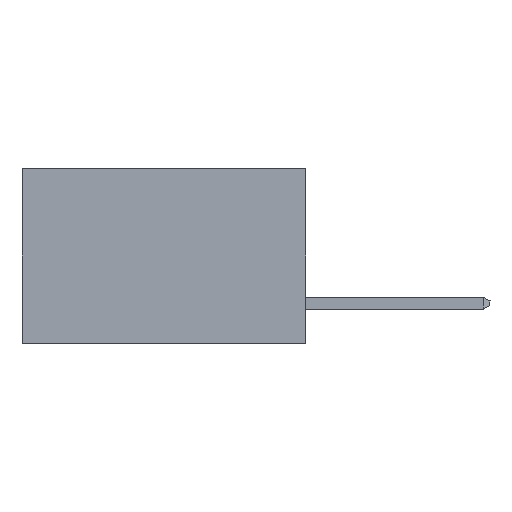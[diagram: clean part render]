
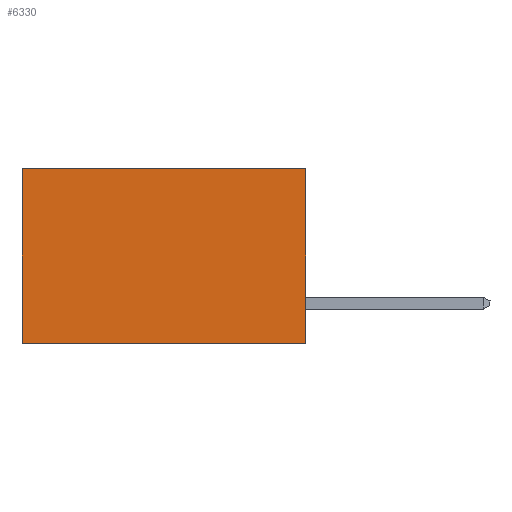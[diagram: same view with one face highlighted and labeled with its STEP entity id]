
A CAD part, left-side view. The second image highlights one B-rep face of the part: STEP entity #6330.
In plain terms, the highlighted planar face has unit normal (-1, 0, 0).
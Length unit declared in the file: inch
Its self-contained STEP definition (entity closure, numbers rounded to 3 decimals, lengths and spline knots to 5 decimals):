
#149 = DIRECTION ( 'NONE',  ( 0., 0., -1. ) ) ;
#611 = CARTESIAN_POINT ( 'NONE',  ( 0.298, 0., 0. ) ) ;
#1782 = LINE ( 'NONE', #18143, #16651 ) ;
#2880 = DIRECTION ( 'NONE',  ( 0., 0., -1. ) ) ;
#3373 = CARTESIAN_POINT ( 'NONE',  ( 0.298, 0.6, -0.37 ) ) ;
#4091 = CARTESIAN_POINT ( 'NONE',  ( 0.298, 0., 0. ) ) ;
#4401 = VERTEX_POINT ( 'NONE', #611 ) ;
#4864 = LINE ( 'NONE', #10929, #11615 ) ;
#5112 = DIRECTION ( 'NONE',  ( 0., 1., 0. ) ) ;
#5606 = CARTESIAN_POINT ( 'NONE',  ( 0.298, 0.6, 0. ) ) ;
#6330 = ADVANCED_FACE ( 'NONE', ( #14099 ), #11244, .F. ) ;
#6711 = DIRECTION ( 'NONE',  ( 0., 0., -1. ) ) ;
#6795 = CARTESIAN_POINT ( 'NONE',  ( 0.298, 0.6, 0. ) ) ;
#7055 = AXIS2_PLACEMENT_3D ( 'NONE', #4091, #17512, #149 ) ;
#7122 = EDGE_CURVE ( 'NONE', #4401, #9740, #12042, .T. ) ;
#7131 = LINE ( 'NONE', #5606, #9578 ) ;
#7983 = VECTOR ( 'NONE', #9682, 39.37008 ) ;
#8058 = VERTEX_POINT ( 'NONE', #3373 ) ;
#9578 = VECTOR ( 'NONE', #2880, 39.37008 ) ;
#9581 = ORIENTED_EDGE ( 'NONE', *, *, #7122, .T. ) ;
#9682 = DIRECTION ( 'NONE',  ( 0., 1., 0. ) ) ;
#9740 = VERTEX_POINT ( 'NONE', #6795 ) ;
#10001 = ORIENTED_EDGE ( 'NONE', *, *, #16575, .T. ) ;
#10256 = EDGE_CURVE ( 'NONE', #4401, #18579, #1782, .T. ) ;
#10929 = CARTESIAN_POINT ( 'NONE',  ( 0.298, 0., -0.37 ) ) ;
#11112 = EDGE_LOOP ( 'NONE', ( #10001, #12701, #12853, #9581 ) ) ;
#11244 = PLANE ( 'NONE',  #7055 ) ;
#11568 = EDGE_CURVE ( 'NONE', #18579, #8058, #4864, .T. ) ;
#11615 = VECTOR ( 'NONE', #5112, 39.37008 ) ;
#12042 = LINE ( 'NONE', #13852, #7983 ) ;
#12701 = ORIENTED_EDGE ( 'NONE', *, *, #11568, .F. ) ;
#12853 = ORIENTED_EDGE ( 'NONE', *, *, #10256, .F. ) ;
#13852 = CARTESIAN_POINT ( 'NONE',  ( 0.298, 0., 0. ) ) ;
#14099 = FACE_OUTER_BOUND ( 'NONE', #11112, .T. ) ;
#16575 = EDGE_CURVE ( 'NONE', #9740, #8058, #7131, .T. ) ;
#16651 = VECTOR ( 'NONE', #6711, 39.37008 ) ;
#17512 = DIRECTION ( 'NONE',  ( 1., 0., 0. ) ) ;
#18143 = CARTESIAN_POINT ( 'NONE',  ( 0.298, 0., 0. ) ) ;
#18579 = VERTEX_POINT ( 'NONE', #18628 ) ;
#18628 = CARTESIAN_POINT ( 'NONE',  ( 0.298, 0., -0.37 ) ) ;
